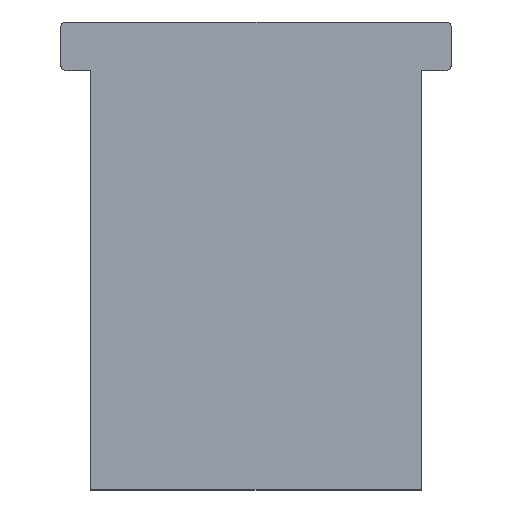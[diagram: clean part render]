
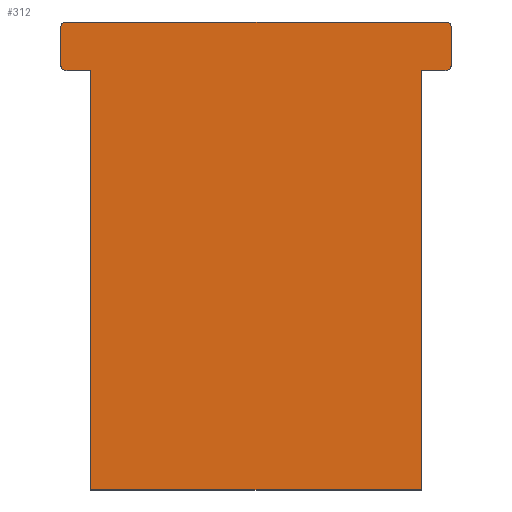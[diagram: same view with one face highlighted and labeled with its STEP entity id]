
A CAD part, top view. The second image highlights one B-rep face of the part: STEP entity #312.
In plain terms, the highlighted planar face has unit normal (0, 0, 1).
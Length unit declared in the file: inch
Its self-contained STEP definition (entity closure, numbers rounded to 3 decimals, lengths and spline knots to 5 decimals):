
#22=PLANE('',#358);
#34=FACE_OUTER_BOUND('',#52,.T.);
#52=EDGE_LOOP('',(#245,#246,#247,#248,#249,#250,#251,#252,#253,#254,#255,
#256));
#69=LINE('',#489,#99);
#78=LINE('',#515,#108);
#80=LINE('',#519,#110);
#81=LINE('',#521,#111);
#82=LINE('',#525,#112);
#83=LINE('',#529,#113);
#84=LINE('',#533,#114);
#85=LINE('',#536,#115);
#99=VECTOR('',#397,0.3937);
#108=VECTOR('',#418,0.3937);
#110=VECTOR('',#422,0.3937);
#111=VECTOR('',#423,0.3937);
#112=VECTOR('',#426,0.3937);
#113=VECTOR('',#429,0.3937);
#114=VECTOR('',#432,0.3937);
#115=VECTOR('',#435,0.3937);
#135=CIRCLE('',#359,0.01);
#136=CIRCLE('',#360,0.01);
#137=CIRCLE('',#361,0.01);
#138=CIRCLE('',#362,0.01);
#147=VERTEX_POINT('',#486);
#148=VERTEX_POINT('',#488);
#159=VERTEX_POINT('',#514);
#160=VERTEX_POINT('',#518);
#161=VERTEX_POINT('',#520);
#162=VERTEX_POINT('',#522);
#163=VERTEX_POINT('',#524);
#164=VERTEX_POINT('',#526);
#165=VERTEX_POINT('',#528);
#166=VERTEX_POINT('',#530);
#167=VERTEX_POINT('',#532);
#168=VERTEX_POINT('',#534);
#179=EDGE_CURVE('',#148,#147,#69,.T.);
#192=EDGE_CURVE('',#148,#159,#78,.T.);
#194=EDGE_CURVE('',#147,#160,#80,.T.);
#195=EDGE_CURVE('',#161,#160,#81,.T.);
#196=EDGE_CURVE('',#162,#161,#135,.T.);
#197=EDGE_CURVE('',#163,#162,#82,.T.);
#198=EDGE_CURVE('',#164,#163,#136,.T.);
#199=EDGE_CURVE('',#165,#164,#83,.T.);
#200=EDGE_CURVE('',#166,#165,#137,.T.);
#201=EDGE_CURVE('',#167,#166,#84,.T.);
#202=EDGE_CURVE('',#168,#167,#138,.T.);
#203=EDGE_CURVE('',#159,#168,#85,.T.);
#245=ORIENTED_EDGE('',*,*,#179,.T.);
#246=ORIENTED_EDGE('',*,*,#194,.T.);
#247=ORIENTED_EDGE('',*,*,#195,.F.);
#248=ORIENTED_EDGE('',*,*,#196,.F.);
#249=ORIENTED_EDGE('',*,*,#197,.F.);
#250=ORIENTED_EDGE('',*,*,#198,.F.);
#251=ORIENTED_EDGE('',*,*,#199,.F.);
#252=ORIENTED_EDGE('',*,*,#200,.F.);
#253=ORIENTED_EDGE('',*,*,#201,.F.);
#254=ORIENTED_EDGE('',*,*,#202,.F.);
#255=ORIENTED_EDGE('',*,*,#203,.F.);
#256=ORIENTED_EDGE('',*,*,#192,.F.);
#312=ADVANCED_FACE('',(#34),#22,.F.);
#358=AXIS2_PLACEMENT_3D('',#517,#420,#421);
#359=AXIS2_PLACEMENT_3D('',#523,#424,#425);
#360=AXIS2_PLACEMENT_3D('',#527,#427,#428);
#361=AXIS2_PLACEMENT_3D('',#531,#430,#431);
#362=AXIS2_PLACEMENT_3D('',#535,#433,#434);
#397=DIRECTION('',(1.,0.,0.));
#418=DIRECTION('',(0.,1.,0.));
#420=DIRECTION('center_axis',(0.,0.,-1.));
#421=DIRECTION('ref_axis',(1.,0.,0.));
#422=DIRECTION('',(0.,1.,0.));
#423=DIRECTION('',(-1.,0.,0.));
#424=DIRECTION('center_axis',(0.,0.,-1.));
#425=DIRECTION('ref_axis',(0.707,-0.707,0.));
#426=DIRECTION('',(0.,-1.,0.));
#427=DIRECTION('center_axis',(0.,0.,-1.));
#428=DIRECTION('ref_axis',(0.707,0.707,0.));
#429=DIRECTION('',(1.,0.,0.));
#430=DIRECTION('center_axis',(0.,0.,-1.));
#431=DIRECTION('ref_axis',(-0.707,0.707,0.));
#432=DIRECTION('',(0.,1.,0.));
#433=DIRECTION('center_axis',(0.,0.,-1.));
#434=DIRECTION('ref_axis',(-0.707,-0.707,0.));
#435=DIRECTION('',(-1.,0.,0.));
#486=CARTESIAN_POINT('',(0.314,-0.44,-2.49283));
#488=CARTESIAN_POINT('',(-0.314,-0.44,-2.49283));
#489=CARTESIAN_POINT('',(-0.10146,-0.44,-2.49283));
#514=CARTESIAN_POINT('',(-0.314,0.35787,-2.49283));
#515=CARTESIAN_POINT('',(-0.314,0.3405,-2.49283));
#517=CARTESIAN_POINT('Origin',(-0.51691,0.45,-2.49283));
#518=CARTESIAN_POINT('',(0.314,0.35787,-2.49283));
#519=CARTESIAN_POINT('',(0.314,-0.88501,-2.49283));
#520=CARTESIAN_POINT('',(0.36156,0.35787,-2.49283));
#521=CARTESIAN_POINT('',(-0.07071,0.35787,-2.49283));
#522=CARTESIAN_POINT('',(0.37156,0.36787,-2.49283));
#523=CARTESIAN_POINT('Origin',(0.36156,0.36787,-2.49283));
#524=CARTESIAN_POINT('',(0.37156,0.44,-2.49283));
#525=CARTESIAN_POINT('',(0.37156,0.45,-2.49283));
#526=CARTESIAN_POINT('',(0.36156,0.45,-2.49283));
#527=CARTESIAN_POINT('Origin',(0.36156,0.44,-2.49283));
#528=CARTESIAN_POINT('',(-0.36156,0.45,-2.49283));
#529=CARTESIAN_POINT('',(-0.06796,0.45,-2.49283));
#530=CARTESIAN_POINT('',(-0.37156,0.44,-2.49283));
#531=CARTESIAN_POINT('Origin',(-0.36156,0.44,-2.49283));
#532=CARTESIAN_POINT('',(-0.37156,0.36787,-2.49283));
#533=CARTESIAN_POINT('',(-0.37156,0.45,-2.49283));
#534=CARTESIAN_POINT('',(-0.36156,0.35787,-2.49283));
#535=CARTESIAN_POINT('Origin',(-0.36156,0.36787,-2.49283));
#536=CARTESIAN_POINT('',(-0.07071,0.35787,-2.49283));
